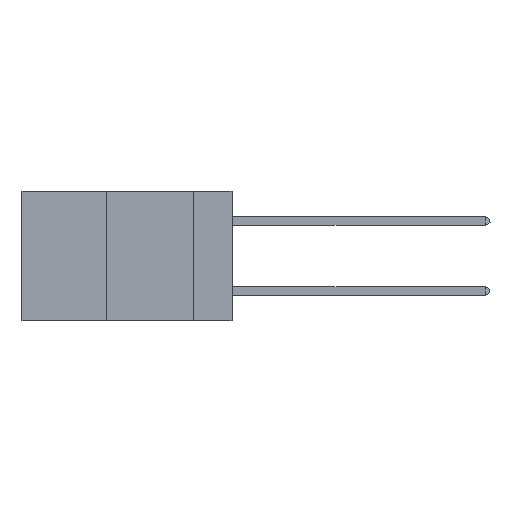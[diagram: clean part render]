
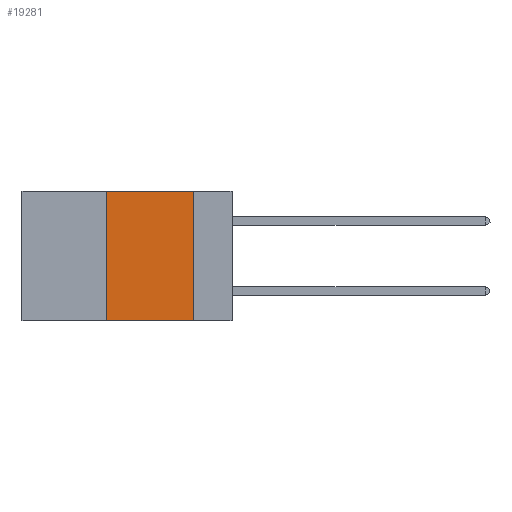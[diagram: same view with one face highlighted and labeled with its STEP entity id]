
A CAD part, left-side view. The second image highlights one B-rep face of the part: STEP entity #19281.
In plain terms, the highlighted planar face has unit normal (-1, 0, 0).
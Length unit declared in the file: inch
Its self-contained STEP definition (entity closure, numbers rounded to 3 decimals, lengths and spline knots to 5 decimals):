
#523 = VERTEX_POINT ( 'NONE', #6009 ) ;
#1142 = DIRECTION ( 'NONE',  ( 0., 0., -1. ) ) ;
#1653 = LINE ( 'NONE', #11609, #6364 ) ;
#2341 = DIRECTION ( 'NONE',  ( 0., 0., -1. ) ) ;
#3826 = CARTESIAN_POINT ( 'NONE',  ( 0., 0.36, -0.37 ) ) ;
#5955 = PLANE ( 'NONE',  #20055 ) ;
#6009 = CARTESIAN_POINT ( 'NONE',  ( 0., 0.11, 0. ) ) ;
#6364 = VECTOR ( 'NONE', #15243, 39.37008 ) ;
#7825 = LINE ( 'NONE', #13088, #9206 ) ;
#8065 = EDGE_CURVE ( 'NONE', #9587, #16532, #1653, .T. ) ;
#8473 = VERTEX_POINT ( 'NONE', #21542 ) ;
#9206 = VECTOR ( 'NONE', #10900, 39.37008 ) ;
#9358 = LINE ( 'NONE', #12220, #14540 ) ;
#9587 = VERTEX_POINT ( 'NONE', #3826 ) ;
#9696 = DIRECTION ( 'NONE',  ( 1., 0., 0. ) ) ;
#10759 = EDGE_CURVE ( 'NONE', #8473, #523, #21522, .T. ) ;
#10808 = ORIENTED_EDGE ( 'NONE', *, *, #13778, .F. ) ;
#10900 = DIRECTION ( 'NONE',  ( 0., 0., 1. ) ) ;
#11337 = CARTESIAN_POINT ( 'NONE',  ( 0., 0.6, 0. ) ) ;
#11446 = DIRECTION ( 'NONE',  ( 0., -1., 0. ) ) ;
#11609 = CARTESIAN_POINT ( 'NONE',  ( 0., 0.6, -0.37 ) ) ;
#12220 = CARTESIAN_POINT ( 'NONE',  ( 0., 0.11, 0. ) ) ;
#12851 = ORIENTED_EDGE ( 'NONE', *, *, #19323, .F. ) ;
#13088 = CARTESIAN_POINT ( 'NONE',  ( 0., 0.36, 0. ) ) ;
#13113 = ORIENTED_EDGE ( 'NONE', *, *, #10759, .F. ) ;
#13778 = EDGE_CURVE ( 'NONE', #523, #16532, #9358, .T. ) ;
#14089 = ORIENTED_EDGE ( 'NONE', *, *, #8065, .T. ) ;
#14540 = VECTOR ( 'NONE', #2341, 39.37008 ) ;
#15243 = DIRECTION ( 'NONE',  ( 0., -1., 0. ) ) ;
#15250 = EDGE_LOOP ( 'NONE', ( #10808, #13113, #12851, #14089 ) ) ;
#16160 = FACE_OUTER_BOUND ( 'NONE', #15250, .T. ) ;
#16532 = VERTEX_POINT ( 'NONE', #17670 ) ;
#17670 = CARTESIAN_POINT ( 'NONE',  ( 0., 0.11, -0.37 ) ) ;
#19281 = ADVANCED_FACE ( 'NONE', ( #16160 ), #5955, .F. ) ;
#19323 = EDGE_CURVE ( 'NONE', #9587, #8473, #7825, .T. ) ;
#19433 = VECTOR ( 'NONE', #11446, 39.37008 ) ;
#19779 = CARTESIAN_POINT ( 'NONE',  ( 0., 0.6, 0. ) ) ;
#20055 = AXIS2_PLACEMENT_3D ( 'NONE', #11337, #9696, #1142 ) ;
#21522 = LINE ( 'NONE', #19779, #19433 ) ;
#21542 = CARTESIAN_POINT ( 'NONE',  ( 0., 0.36, 0. ) ) ;
